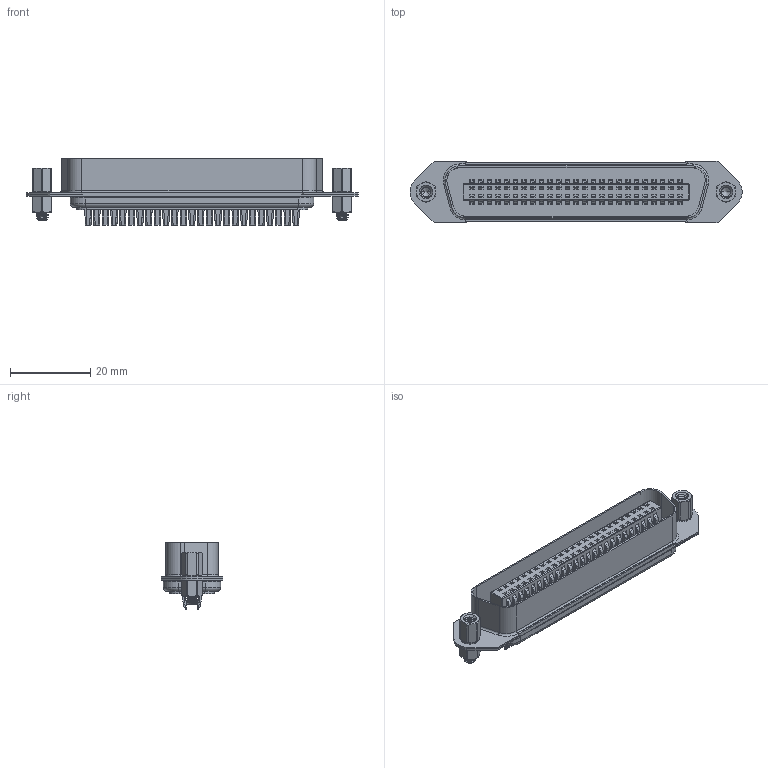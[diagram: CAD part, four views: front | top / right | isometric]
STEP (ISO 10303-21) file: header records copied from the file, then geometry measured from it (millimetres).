
FILE_DESCRIPTION (( 'STEP AP203' ), '1' );
FILE_NAME ('B57-150-622-F02.STEP', '2020-06-24T12:45:28', ( '' ), ( '' ), 'SwSTEP 2.0', 'SolidWorks 2020', '' );
FILE_SCHEMA (( 'CONFIG_CONTROL_DESIGN' ));
Length unit declared in the file: millimetre
Products named in the file (7): B57 Hex Standoff; B57 Front Shell MALE_50 Position UP; B57-150-622-F02; B57 Back Shell_50 Position; B57 Rivet_STR HEX STANDOFF; B57 Housing Insert MALE_50 Position UP; B57 Contacts MALE_50 Position SOLDER
Assembly tree (8 placements, depth 2):
  B57-150-622-F02
    B57 Back Shell_50 Position
    B57 Rivet_STR HEX STANDOFF  x2
    B57 Housing Insert MALE_50 Position UP
    B57 Front Shell MALE_50 Position UP
    B57 Contacts MALE_50 Position SOLDER
    B57 Hex Standoff  x2
Bounding box: 82.83 x 15.3 x 16.57 mm (x, y, z)
Volume: 6238.9 mm3; surface area: 15439 mm2
Topology: 57 solids, 57 shells, 5467 faces, 15529 edges, 9880 vertices
Faces by surface type: plane 3809, cylinder 1344, sphere 204, cone 62, torus 30, bspline 18
Entity records: 175036 total; most frequent: CARTESIAN_POINT 36986, ORIENTED_EDGE 29954, DIRECTION 26991, EDGE_CURVE 14977, LINE 11851, VECTOR 11851, VERTEX_POINT 9656, AXIS2_PLACEMENT_3D 7570
